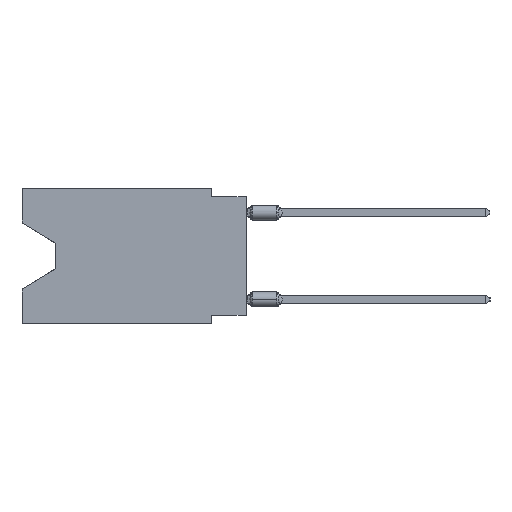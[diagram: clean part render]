
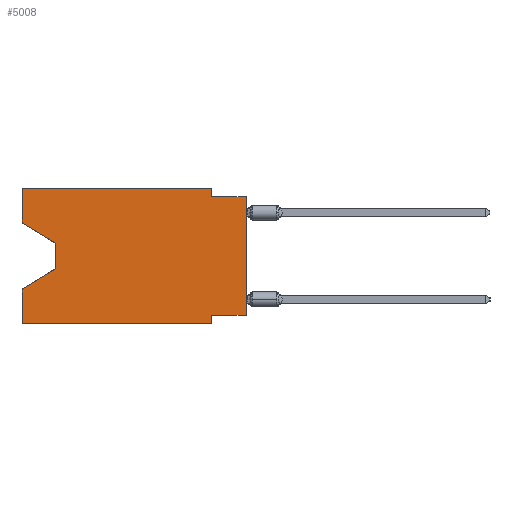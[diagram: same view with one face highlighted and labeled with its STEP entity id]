
A CAD part, left-side view. The second image highlights one B-rep face of the part: STEP entity #5008.
In plain terms, the highlighted planar face has unit normal (-1, 0, 0).
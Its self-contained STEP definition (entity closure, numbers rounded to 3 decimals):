
#608 = LINE ( 'NONE', #60439, #17148 ) ;
#963 = EDGE_LOOP ( 'NONE', ( #51089, #28497, #53417, #13863, #51440, #49950, #59217, #10061, #21540, #43939, #3164, #13393 ) ) ;
#1679 = VECTOR ( 'NONE', #46036, 1000. ) ;
#2137 = VECTOR ( 'NONE', #19040, 1000. ) ;
#3164 = ORIENTED_EDGE ( 'NONE', *, *, #8502, .F. ) ;
#3471 = CARTESIAN_POINT ( 'NONE',  ( 0., 13.97, -5.893 ) ) ;
#4266 = CARTESIAN_POINT ( 'NONE',  ( 0., 0., -0.635 ) ) ;
#5008 = ADVANCED_FACE ( 'NONE', ( #25438 ), #54269, .F. ) ;
#5027 = CARTESIAN_POINT ( 'NONE',  ( 0., 0., 0. ) ) ;
#5049 = DIRECTION ( 'NONE',  ( 0., 1., 0. ) ) ;
#6040 = VECTOR ( 'NONE', #5049, 1000. ) ;
#6545 = EDGE_CURVE ( 'NONE', #17884, #36018, #47090, .T. ) ;
#6771 = VERTEX_POINT ( 'NONE', #3471 ) ;
#8502 = EDGE_CURVE ( 'NONE', #51154, #23519, #10129, .T. ) ;
#8581 = LINE ( 'NONE', #60111, #27768 ) ;
#9024 = LINE ( 'NONE', #13939, #27647 ) ;
#9127 = VECTOR ( 'NONE', #25288, 1000. ) ;
#9635 = DIRECTION ( 'NONE',  ( 0., 0., 1. ) ) ;
#10061 = ORIENTED_EDGE ( 'NONE', *, *, #28509, .T. ) ;
#10129 = LINE ( 'NONE', #60445, #2137 ) ;
#10531 = VERTEX_POINT ( 'NONE', #41740 ) ;
#10565 = EDGE_CURVE ( 'NONE', #11159, #40593, #608, .T. ) ;
#11159 = VERTEX_POINT ( 'NONE', #11568 ) ;
#11568 = CARTESIAN_POINT ( 'NONE',  ( 0., 16.383, -9.906 ) ) ;
#12934 = VECTOR ( 'NONE', #50782, 1000. ) ;
#13393 = ORIENTED_EDGE ( 'NONE', *, *, #16610, .F. ) ;
#13566 = VECTOR ( 'NONE', #17178, 1000. ) ;
#13863 = ORIENTED_EDGE ( 'NONE', *, *, #31627, .F. ) ;
#13939 = CARTESIAN_POINT ( 'NONE',  ( 0., 2.54, 0. ) ) ;
#15667 = LINE ( 'NONE', #19370, #60529 ) ;
#16610 = EDGE_CURVE ( 'NONE', #49770, #51154, #59238, .T. ) ;
#16876 = LINE ( 'NONE', #59792, #13566 ) ;
#17148 = VECTOR ( 'NONE', #51861, 1000. ) ;
#17178 = DIRECTION ( 'NONE',  ( 0., 0., -1. ) ) ;
#17884 = VERTEX_POINT ( 'NONE', #60643 ) ;
#18542 = LINE ( 'NONE', #22850, #12934 ) ;
#18847 = LINE ( 'NONE', #5027, #29621 ) ;
#19040 = DIRECTION ( 'NONE',  ( 0., -1., 0. ) ) ;
#19370 = CARTESIAN_POINT ( 'NONE',  ( 0., 0., -0.635 ) ) ;
#21374 = CARTESIAN_POINT ( 'NONE',  ( 0., 2.54, -9.906 ) ) ;
#21540 = ORIENTED_EDGE ( 'NONE', *, *, #59950, .F. ) ;
#21846 = VERTEX_POINT ( 'NONE', #4266 ) ;
#22850 = CARTESIAN_POINT ( 'NONE',  ( 0., 2.54, -9.906 ) ) ;
#23519 = VERTEX_POINT ( 'NONE', #42547 ) ;
#23761 = EDGE_CURVE ( 'NONE', #36018, #40593, #18542, .T. ) ;
#24297 = CARTESIAN_POINT ( 'NONE',  ( 0., 16.383, 0. ) ) ;
#25288 = DIRECTION ( 'NONE',  ( 0., 0.855, -0.519 ) ) ;
#25438 = FACE_OUTER_BOUND ( 'NONE', #963, .T. ) ;
#26291 = CARTESIAN_POINT ( 'NONE',  ( 0., 16.383, -2.546 ) ) ;
#27647 = VECTOR ( 'NONE', #46462, 1000. ) ;
#27768 = VECTOR ( 'NONE', #36804, 1000. ) ;
#28437 = EDGE_CURVE ( 'NONE', #23519, #10531, #9024, .T. ) ;
#28497 = ORIENTED_EDGE ( 'NONE', *, *, #44446, .T. ) ;
#28509 = EDGE_CURVE ( 'NONE', #17884, #21846, #18847, .T. ) ;
#29621 = VECTOR ( 'NONE', #9635, 1000. ) ;
#30640 = DIRECTION ( 'NONE',  ( 1., 0., 0. ) ) ;
#31627 = EDGE_CURVE ( 'NONE', #11159, #44360, #8581, .T. ) ;
#32221 = CARTESIAN_POINT ( 'NONE',  ( 0., 16.383, 0. ) ) ;
#33544 = VERTEX_POINT ( 'NONE', #53378 ) ;
#35401 = LINE ( 'NONE', #58099, #9127 ) ;
#35507 = LINE ( 'NONE', #26291, #50660 ) ;
#36018 = VERTEX_POINT ( 'NONE', #36800 ) ;
#36800 = CARTESIAN_POINT ( 'NONE',  ( 0., 2.54, -9.271 ) ) ;
#36804 = DIRECTION ( 'NONE',  ( 0., 0., 1. ) ) ;
#38975 = DIRECTION ( 'NONE',  ( 0., -1., 0. ) ) ;
#39198 = DIRECTION ( 'NONE',  ( 0., -0.855, -0.519 ) ) ;
#40464 = DIRECTION ( 'NONE',  ( 0., 0., -1. ) ) ;
#40593 = VERTEX_POINT ( 'NONE', #21374 ) ;
#41740 = CARTESIAN_POINT ( 'NONE',  ( 0., 2.54, -0.635 ) ) ;
#42547 = CARTESIAN_POINT ( 'NONE',  ( 0., 2.54, 0. ) ) ;
#43279 = CARTESIAN_POINT ( 'NONE',  ( 0., 16.383, -7.36 ) ) ;
#43939 = ORIENTED_EDGE ( 'NONE', *, *, #28437, .F. ) ;
#44146 = CARTESIAN_POINT ( 'NONE',  ( 0., 16.383, 0. ) ) ;
#44360 = VERTEX_POINT ( 'NONE', #43279 ) ;
#44446 = EDGE_CURVE ( 'NONE', #33544, #6771, #16876, .T. ) ;
#46036 = DIRECTION ( 'NONE',  ( 0., 0., 1. ) ) ;
#46462 = DIRECTION ( 'NONE',  ( 0., 0., -1. ) ) ;
#47090 = LINE ( 'NONE', #52596, #6040 ) ;
#49770 = VERTEX_POINT ( 'NONE', #52904 ) ;
#49950 = ORIENTED_EDGE ( 'NONE', *, *, #23761, .F. ) ;
#50660 = VECTOR ( 'NONE', #39198, 1000. ) ;
#50782 = DIRECTION ( 'NONE',  ( 0., 0., -1. ) ) ;
#51089 = ORIENTED_EDGE ( 'NONE', *, *, #59250, .T. ) ;
#51154 = VERTEX_POINT ( 'NONE', #24297 ) ;
#51440 = ORIENTED_EDGE ( 'NONE', *, *, #10565, .T. ) ;
#51861 = DIRECTION ( 'NONE',  ( 0., -1., 0. ) ) ;
#52143 = EDGE_CURVE ( 'NONE', #6771, #44360, #35401, .T. ) ;
#52596 = CARTESIAN_POINT ( 'NONE',  ( 0., 0., -9.271 ) ) ;
#52904 = CARTESIAN_POINT ( 'NONE',  ( 0., 16.383, -2.546 ) ) ;
#53378 = CARTESIAN_POINT ( 'NONE',  ( 0., 13.97, -4.013 ) ) ;
#53417 = ORIENTED_EDGE ( 'NONE', *, *, #52143, .T. ) ;
#54269 = PLANE ( 'NONE',  #54882 ) ;
#54882 = AXIS2_PLACEMENT_3D ( 'NONE', #44146, #30640, #40464 ) ;
#58099 = CARTESIAN_POINT ( 'NONE',  ( 0., 13.97, -5.893 ) ) ;
#59217 = ORIENTED_EDGE ( 'NONE', *, *, #6545, .F. ) ;
#59238 = LINE ( 'NONE', #32221, #1679 ) ;
#59250 = EDGE_CURVE ( 'NONE', #49770, #33544, #35507, .T. ) ;
#59792 = CARTESIAN_POINT ( 'NONE',  ( 0., 13.97, -4.013 ) ) ;
#59950 = EDGE_CURVE ( 'NONE', #10531, #21846, #15667, .T. ) ;
#60111 = CARTESIAN_POINT ( 'NONE',  ( 0., 16.383, 0. ) ) ;
#60439 = CARTESIAN_POINT ( 'NONE',  ( 0., 16.383, -9.906 ) ) ;
#60445 = CARTESIAN_POINT ( 'NONE',  ( 0., 16.383, 0. ) ) ;
#60529 = VECTOR ( 'NONE', #38975, 1000. ) ;
#60643 = CARTESIAN_POINT ( 'NONE',  ( 0., 0., -9.271 ) ) ;
